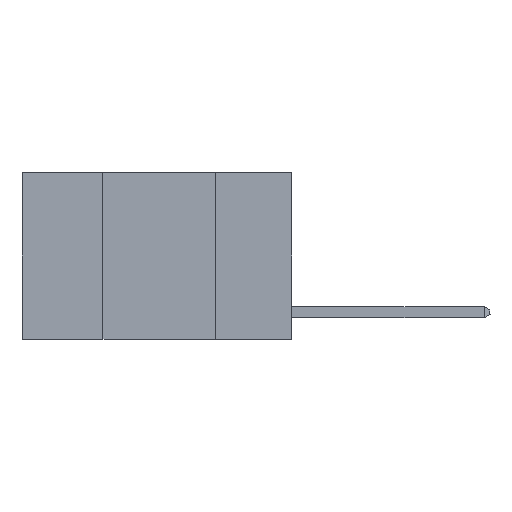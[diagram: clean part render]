
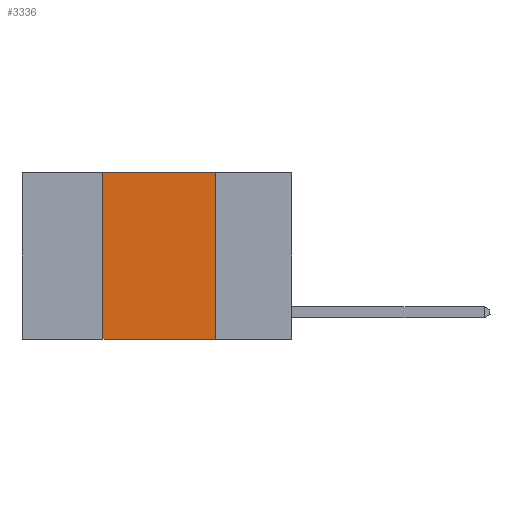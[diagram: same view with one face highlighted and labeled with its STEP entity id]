
A CAD part, left-side view. The second image highlights one B-rep face of the part: STEP entity #3336.
In plain terms, the highlighted planar face has unit normal (-1, 0, 0).
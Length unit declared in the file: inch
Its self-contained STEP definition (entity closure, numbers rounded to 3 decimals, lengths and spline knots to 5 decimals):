
#262 = CARTESIAN_POINT ( 'NONE',  ( 0., 0.6, 0. ) ) ;
#890 = CARTESIAN_POINT ( 'NONE',  ( 0., 0.17, 0. ) ) ;
#1259 = LINE ( 'NONE', #7511, #14719 ) ;
#1989 = DIRECTION ( 'NONE',  ( 0., -1., 0. ) ) ;
#2099 = VERTEX_POINT ( 'NONE', #17842 ) ;
#2361 = PLANE ( 'NONE',  #6103 ) ;
#2435 = CARTESIAN_POINT ( 'NONE',  ( 0., 0.6, 0. ) ) ;
#2681 = VERTEX_POINT ( 'NONE', #890 ) ;
#3336 = ADVANCED_FACE ( 'NONE', ( #21859 ), #2361, .F. ) ;
#3518 = ORIENTED_EDGE ( 'NONE', *, *, #11630, .F. ) ;
#4430 = CARTESIAN_POINT ( 'NONE',  ( 0., 0.42, 0. ) ) ;
#5783 = VECTOR ( 'NONE', #20129, 39.37008 ) ;
#5867 = DIRECTION ( 'NONE',  ( 1., 0., 0. ) ) ;
#6103 = AXIS2_PLACEMENT_3D ( 'NONE', #2435, #5867, #17559 ) ;
#6723 = ORIENTED_EDGE ( 'NONE', *, *, #19612, .F. ) ;
#7010 = EDGE_LOOP ( 'NONE', ( #3518, #6723, #11223, #11278 ) ) ;
#7511 = CARTESIAN_POINT ( 'NONE',  ( 0., 0.42, 0. ) ) ;
#8022 = CARTESIAN_POINT ( 'NONE',  ( 0., 0.6, -0.37 ) ) ;
#10133 = CARTESIAN_POINT ( 'NONE',  ( 0., 0.17, 0. ) ) ;
#11041 = CARTESIAN_POINT ( 'NONE',  ( 0., 0.17, -0.37 ) ) ;
#11223 = ORIENTED_EDGE ( 'NONE', *, *, #11236, .F. ) ;
#11236 = EDGE_CURVE ( 'NONE', #2099, #14614, #1259, .T. ) ;
#11278 = ORIENTED_EDGE ( 'NONE', *, *, #18099, .T. ) ;
#11630 = EDGE_CURVE ( 'NONE', #2681, #21709, #18630, .T. ) ;
#12277 = LINE ( 'NONE', #262, #16164 ) ;
#14614 = VERTEX_POINT ( 'NONE', #4430 ) ;
#14719 = VECTOR ( 'NONE', #17485, 39.37008 ) ;
#16164 = VECTOR ( 'NONE', #1989, 39.37008 ) ;
#17042 = LINE ( 'NONE', #8022, #20979 ) ;
#17485 = DIRECTION ( 'NONE',  ( 0., 0., 1. ) ) ;
#17559 = DIRECTION ( 'NONE',  ( 0., 0., -1. ) ) ;
#17842 = CARTESIAN_POINT ( 'NONE',  ( 0., 0.42, -0.37 ) ) ;
#18099 = EDGE_CURVE ( 'NONE', #2099, #21709, #17042, .T. ) ;
#18630 = LINE ( 'NONE', #10133, #5783 ) ;
#19612 = EDGE_CURVE ( 'NONE', #14614, #2681, #12277, .T. ) ;
#20129 = DIRECTION ( 'NONE',  ( 0., 0., -1. ) ) ;
#20979 = VECTOR ( 'NONE', #21380, 39.37008 ) ;
#21380 = DIRECTION ( 'NONE',  ( 0., -1., 0. ) ) ;
#21709 = VERTEX_POINT ( 'NONE', #11041 ) ;
#21859 = FACE_OUTER_BOUND ( 'NONE', #7010, .T. ) ;
